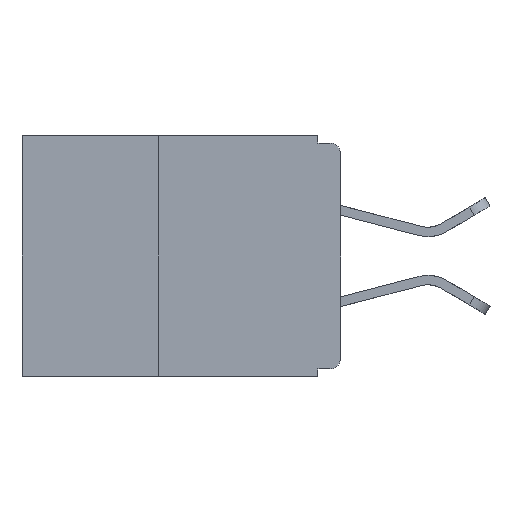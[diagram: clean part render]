
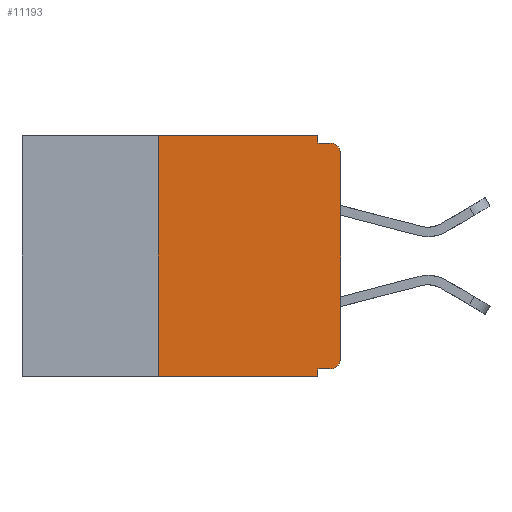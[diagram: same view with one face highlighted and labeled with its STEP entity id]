
A CAD part, left-side view. The second image highlights one B-rep face of the part: STEP entity #11193.
In plain terms, the highlighted planar face has unit normal (-1, 0, 0).
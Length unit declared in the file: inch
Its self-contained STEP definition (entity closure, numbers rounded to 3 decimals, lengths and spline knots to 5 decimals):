
#77 = ORIENTED_EDGE ( 'NONE', *, *, #3826, .F. ) ;
#406 = ORIENTED_EDGE ( 'NONE', *, *, #10408, .F. ) ;
#428 = DIRECTION ( 'NONE',  ( 0., 0., -1. ) ) ;
#788 = LINE ( 'NONE', #7804, #5419 ) ;
#1159 = DIRECTION ( 'NONE',  ( 0., -1., 0. ) ) ;
#1176 = VERTEX_POINT ( 'NONE', #7396 ) ;
#1210 = VERTEX_POINT ( 'NONE', #7536 ) ;
#1217 = VECTOR ( 'NONE', #4247, 39.37008 ) ;
#1223 = VERTEX_POINT ( 'NONE', #1937 ) ;
#1519 = LINE ( 'NONE', #6326, #1217 ) ;
#1614 = EDGE_CURVE ( 'NONE', #1744, #4336, #3440, .T. ) ;
#1693 = FACE_OUTER_BOUND ( 'NONE', #5598, .T. ) ;
#1744 = VERTEX_POINT ( 'NONE', #7370 ) ;
#1937 = CARTESIAN_POINT ( 'NONE',  ( 0., 0.015, -0.01 ) ) ;
#2312 = ORIENTED_EDGE ( 'NONE', *, *, #2741, .F. ) ;
#2625 = EDGE_CURVE ( 'NONE', #4336, #1176, #9779, .T. ) ;
#2741 = EDGE_CURVE ( 'NONE', #10217, #1744, #8746, .T. ) ;
#2848 = CARTESIAN_POINT ( 'NONE',  ( 0., 0., -0.305 ) ) ;
#2884 = ORIENTED_EDGE ( 'NONE', *, *, #10933, .T. ) ;
#2982 = CARTESIAN_POINT ( 'NONE',  ( 0., 0.031, 0. ) ) ;
#3129 = VECTOR ( 'NONE', #5770, 39.37008 ) ;
#3265 = CARTESIAN_POINT ( 'NONE',  ( 0., 0.437, 0. ) ) ;
#3339 = CARTESIAN_POINT ( 'NONE',  ( 0., 0.437, 0. ) ) ;
#3436 = AXIS2_PLACEMENT_3D ( 'NONE', #3941, #10078, #4876 ) ;
#3440 = LINE ( 'NONE', #3265, #7744 ) ;
#3581 = ORIENTED_EDGE ( 'NONE', *, *, #9044, .T. ) ;
#3825 = AXIS2_PLACEMENT_3D ( 'NONE', #3339, #9546, #4266 ) ;
#3826 = EDGE_CURVE ( 'NONE', #7400, #7817, #9745, .T. ) ;
#3870 = ORIENTED_EDGE ( 'NONE', *, *, #2625, .F. ) ;
#3897 = EDGE_CURVE ( 'NONE', #10217, #7817, #1519, .T. ) ;
#3941 = CARTESIAN_POINT ( 'NONE',  ( 0., 0.015, -0.305 ) ) ;
#3997 = LINE ( 'NONE', #9347, #8762 ) ;
#4247 = DIRECTION ( 'NONE',  ( 0., -1., 0. ) ) ;
#4266 = DIRECTION ( 'NONE',  ( 0., 0., -1. ) ) ;
#4267 = DIRECTION ( 'NONE',  ( 0., 0., -1. ) ) ;
#4336 = VERTEX_POINT ( 'NONE', #2982 ) ;
#4472 = CARTESIAN_POINT ( 'NONE',  ( 0., 0.031, -0.33 ) ) ;
#4567 = VECTOR ( 'NONE', #4267, 39.37008 ) ;
#4876 = DIRECTION ( 'NONE',  ( 0., 0., -1. ) ) ;
#4969 = CARTESIAN_POINT ( 'NONE',  ( 0., 0.015, -0.32 ) ) ;
#5004 = CIRCLE ( 'NONE', #8854, 0.015 ) ;
#5096 = DIRECTION ( 'NONE',  ( 0., 1., 0. ) ) ;
#5406 = DIRECTION ( 'NONE',  ( 0., -1., 0. ) ) ;
#5419 = VECTOR ( 'NONE', #5096, 39.37008 ) ;
#5598 = EDGE_LOOP ( 'NONE', ( #3581, #8384, #10556, #3870, #6346, #2312, #7198, #77, #406, #2884 ) ) ;
#5674 = CARTESIAN_POINT ( 'NONE',  ( 0., 0.031, 0. ) ) ;
#5755 = CARTESIAN_POINT ( 'NONE',  ( 0., 0., -0.01 ) ) ;
#5770 = DIRECTION ( 'NONE',  ( 0., 0., 1. ) ) ;
#5800 = CARTESIAN_POINT ( 'NONE',  ( 0., 0.25, -0.33 ) ) ;
#5971 = DIRECTION ( 'NONE',  ( -1., 0., 0. ) ) ;
#6159 = CIRCLE ( 'NONE', #3436, 0.015 ) ;
#6326 = CARTESIAN_POINT ( 'NONE',  ( 0., 0.437, -0.33 ) ) ;
#6346 = ORIENTED_EDGE ( 'NONE', *, *, #1614, .F. ) ;
#6465 = LINE ( 'NONE', #5755, #10660 ) ;
#6827 = DIRECTION ( 'NONE',  ( 0., 0., 1. ) ) ;
#7198 = ORIENTED_EDGE ( 'NONE', *, *, #3897, .T. ) ;
#7370 = CARTESIAN_POINT ( 'NONE',  ( 0., 0.25, 0. ) ) ;
#7396 = CARTESIAN_POINT ( 'NONE',  ( 0., 0.031, -0.01 ) ) ;
#7400 = VERTEX_POINT ( 'NONE', #9999 ) ;
#7536 = CARTESIAN_POINT ( 'NONE',  ( 0., 0., -0.025 ) ) ;
#7576 = CARTESIAN_POINT ( 'NONE',  ( 0., 0.25, -0.33 ) ) ;
#7744 = VECTOR ( 'NONE', #5406, 39.37008 ) ;
#7804 = CARTESIAN_POINT ( 'NONE',  ( 0., 0., -0.32 ) ) ;
#7817 = VERTEX_POINT ( 'NONE', #8198 ) ;
#7851 = VERTEX_POINT ( 'NONE', #2848 ) ;
#8198 = CARTESIAN_POINT ( 'NONE',  ( 0., 0.031, -0.33 ) ) ;
#8384 = ORIENTED_EDGE ( 'NONE', *, *, #11077, .T. ) ;
#8553 = VERTEX_POINT ( 'NONE', #4969 ) ;
#8746 = LINE ( 'NONE', #5800, #3129 ) ;
#8762 = VECTOR ( 'NONE', #6827, 39.37008 ) ;
#8854 = AXIS2_PLACEMENT_3D ( 'NONE', #11027, #5971, #428 ) ;
#9044 = EDGE_CURVE ( 'NONE', #7851, #1210, #3997, .T. ) ;
#9066 = DIRECTION ( 'NONE',  ( 0., 0., -1. ) ) ;
#9347 = CARTESIAN_POINT ( 'NONE',  ( 0., 0., 0. ) ) ;
#9534 = EDGE_CURVE ( 'NONE', #1176, #1223, #6465, .T. ) ;
#9546 = DIRECTION ( 'NONE',  ( 1., 0., 0. ) ) ;
#9745 = LINE ( 'NONE', #4472, #11369 ) ;
#9779 = LINE ( 'NONE', #5674, #4567 ) ;
#9999 = CARTESIAN_POINT ( 'NONE',  ( 0., 0.031, -0.32 ) ) ;
#10078 = DIRECTION ( 'NONE',  ( -1., 0., 0. ) ) ;
#10217 = VERTEX_POINT ( 'NONE', #7576 ) ;
#10408 = EDGE_CURVE ( 'NONE', #8553, #7400, #788, .T. ) ;
#10556 = ORIENTED_EDGE ( 'NONE', *, *, #9534, .F. ) ;
#10660 = VECTOR ( 'NONE', #1159, 39.37008 ) ;
#10933 = EDGE_CURVE ( 'NONE', #8553, #7851, #6159, .T. ) ;
#11027 = CARTESIAN_POINT ( 'NONE',  ( 0., 0.015, -0.025 ) ) ;
#11077 = EDGE_CURVE ( 'NONE', #1210, #1223, #5004, .T. ) ;
#11131 = PLANE ( 'NONE',  #3825 ) ;
#11193 = ADVANCED_FACE ( 'NONE', ( #1693 ), #11131, .F. ) ;
#11369 = VECTOR ( 'NONE', #9066, 39.37008 ) ;
